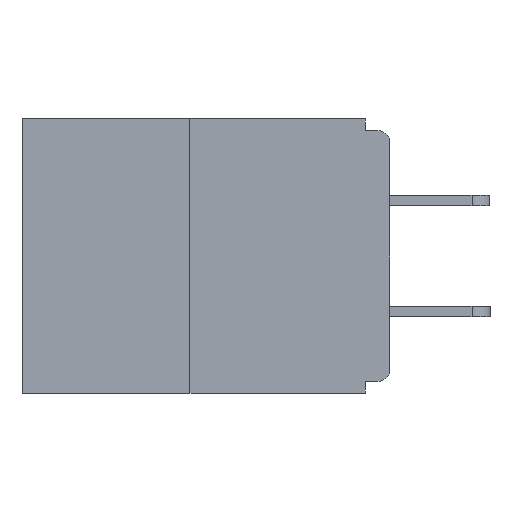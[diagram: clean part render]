
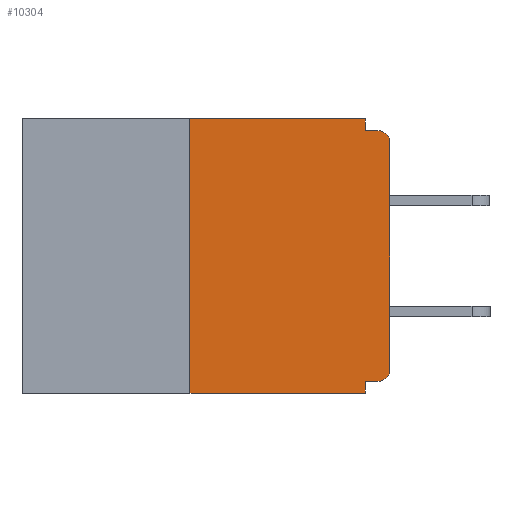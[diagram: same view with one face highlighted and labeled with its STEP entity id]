
A CAD part, left-side view. The second image highlights one B-rep face of the part: STEP entity #10304.
In plain terms, the highlighted planar face has unit normal (-1, 0, 0).
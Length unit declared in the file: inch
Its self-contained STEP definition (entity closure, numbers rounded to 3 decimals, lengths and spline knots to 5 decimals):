
#172 = CARTESIAN_POINT ( 'NONE',  ( 0., 0.25, 0. ) ) ;
#499 = EDGE_CURVE ( 'NONE', #18457, #21759, #11031, .T. ) ;
#586 = CARTESIAN_POINT ( 'NONE',  ( 0., 0.031, 0. ) ) ;
#733 = ORIENTED_EDGE ( 'NONE', *, *, #3186, .T. ) ;
#910 = LINE ( 'NONE', #6174, #18029 ) ;
#940 = DIRECTION ( 'NONE',  ( 0., -1., 0. ) ) ;
#1037 = VERTEX_POINT ( 'NONE', #5647 ) ;
#1962 = LINE ( 'NONE', #22350, #12063 ) ;
#1968 = VERTEX_POINT ( 'NONE', #5962 ) ;
#2229 = CARTESIAN_POINT ( 'NONE',  ( 0., 0.25, -0.343 ) ) ;
#3124 = EDGE_CURVE ( 'NONE', #4434, #1037, #19888, .T. ) ;
#3186 = EDGE_CURVE ( 'NONE', #19924, #1037, #22337, .T. ) ;
#3203 = ORIENTED_EDGE ( 'NONE', *, *, #18955, .T. ) ;
#3213 = CARTESIAN_POINT ( 'NONE',  ( 0., 0.015, -0.015 ) ) ;
#3236 = CARTESIAN_POINT ( 'NONE',  ( 0., 0.46, 0. ) ) ;
#3312 = ORIENTED_EDGE ( 'NONE', *, *, #21635, .F. ) ;
#3404 = CARTESIAN_POINT ( 'NONE',  ( 0., 0.031, 0. ) ) ;
#3610 = DIRECTION ( 'NONE',  ( 0., 0., -1. ) ) ;
#3666 = DIRECTION ( 'NONE',  ( 0., 0., 1. ) ) ;
#4434 = VERTEX_POINT ( 'NONE', #6158 ) ;
#4980 = DIRECTION ( 'NONE',  ( 0., 0., 1. ) ) ;
#5052 = DIRECTION ( 'NONE',  ( 0., 0., -1. ) ) ;
#5203 = DIRECTION ( 'NONE',  ( 0., 0., -1. ) ) ;
#5257 = CARTESIAN_POINT ( 'NONE',  ( 0., 0.015, -0.313 ) ) ;
#5304 = CARTESIAN_POINT ( 'NONE',  ( 0., 0.031, -0.015 ) ) ;
#5647 = CARTESIAN_POINT ( 'NONE',  ( 0., 0.031, -0.343 ) ) ;
#5962 = CARTESIAN_POINT ( 'NONE',  ( 0., 0., -0.313 ) ) ;
#6158 = CARTESIAN_POINT ( 'NONE',  ( 0., 0.031, -0.328 ) ) ;
#6174 = CARTESIAN_POINT ( 'NONE',  ( 0., 0., -0.015 ) ) ;
#6202 = EDGE_CURVE ( 'NONE', #12176, #1968, #8541, .T. ) ;
#6522 = DIRECTION ( 'NONE',  ( -1., 0., 0. ) ) ;
#7012 = CARTESIAN_POINT ( 'NONE',  ( 0., 0., -0.03 ) ) ;
#7045 = DIRECTION ( 'NONE',  ( 1., 0., 0. ) ) ;
#8274 = EDGE_LOOP ( 'NONE', ( #14241, #15948, #733, #13945, #16941, #13226, #18513, #3203, #3312, #21714 ) ) ;
#8541 = CIRCLE ( 'NONE', #15585, 0.015 ) ;
#9002 = VECTOR ( 'NONE', #3666, 39.37008 ) ;
#9113 = VECTOR ( 'NONE', #12593, 39.37008 ) ;
#9220 = FACE_OUTER_BOUND ( 'NONE', #8274, .T. ) ;
#9306 = VECTOR ( 'NONE', #5203, 39.37008 ) ;
#9502 = CARTESIAN_POINT ( 'NONE',  ( 0., 0.46, -0.343 ) ) ;
#10304 = ADVANCED_FACE ( 'NONE', ( #9220 ), #11923, .F. ) ;
#10597 = VERTEX_POINT ( 'NONE', #7012 ) ;
#10696 = LINE ( 'NONE', #15872, #16679 ) ;
#11031 = LINE ( 'NONE', #586, #9113 ) ;
#11128 = CIRCLE ( 'NONE', #17450, 0.015 ) ;
#11409 = DIRECTION ( 'NONE',  ( 0., -1., 0. ) ) ;
#11770 = CARTESIAN_POINT ( 'NONE',  ( 0., 0., 0. ) ) ;
#11923 = PLANE ( 'NONE',  #18122 ) ;
#12063 = VECTOR ( 'NONE', #12115, 39.37008 ) ;
#12115 = DIRECTION ( 'NONE',  ( 0., 1., 0. ) ) ;
#12176 = VERTEX_POINT ( 'NONE', #12956 ) ;
#12491 = CARTESIAN_POINT ( 'NONE',  ( 0., 0.25, 0. ) ) ;
#12593 = DIRECTION ( 'NONE',  ( 0., 0., -1. ) ) ;
#12677 = LINE ( 'NONE', #11770, #20739 ) ;
#12759 = EDGE_CURVE ( 'NONE', #19924, #14581, #20939, .T. ) ;
#12956 = CARTESIAN_POINT ( 'NONE',  ( 0., 0.015, -0.328 ) ) ;
#13226 = ORIENTED_EDGE ( 'NONE', *, *, #6202, .T. ) ;
#13945 = ORIENTED_EDGE ( 'NONE', *, *, #3124, .F. ) ;
#14241 = ORIENTED_EDGE ( 'NONE', *, *, #18108, .F. ) ;
#14581 = VERTEX_POINT ( 'NONE', #12491 ) ;
#15316 = CARTESIAN_POINT ( 'NONE',  ( 0., 0.015, -0.03 ) ) ;
#15585 = AXIS2_PLACEMENT_3D ( 'NONE', #5257, #15679, #17448 ) ;
#15679 = DIRECTION ( 'NONE',  ( -1., 0., 0. ) ) ;
#15872 = CARTESIAN_POINT ( 'NONE',  ( 0., 0.46, 0. ) ) ;
#15948 = ORIENTED_EDGE ( 'NONE', *, *, #12759, .F. ) ;
#16679 = VECTOR ( 'NONE', #17856, 39.37008 ) ;
#16941 = ORIENTED_EDGE ( 'NONE', *, *, #21707, .F. ) ;
#17448 = DIRECTION ( 'NONE',  ( 0., 0., -1. ) ) ;
#17450 = AXIS2_PLACEMENT_3D ( 'NONE', #15316, #6522, #5052 ) ;
#17608 = CARTESIAN_POINT ( 'NONE',  ( 0., 0.031, -0.343 ) ) ;
#17856 = DIRECTION ( 'NONE',  ( 0., -1., 0. ) ) ;
#18029 = VECTOR ( 'NONE', #11409, 39.37008 ) ;
#18108 = EDGE_CURVE ( 'NONE', #14581, #18457, #10696, .T. ) ;
#18122 = AXIS2_PLACEMENT_3D ( 'NONE', #3236, #7045, #3610 ) ;
#18457 = VERTEX_POINT ( 'NONE', #3404 ) ;
#18513 = ORIENTED_EDGE ( 'NONE', *, *, #18960, .T. ) ;
#18955 = EDGE_CURVE ( 'NONE', #10597, #22397, #11128, .T. ) ;
#18960 = EDGE_CURVE ( 'NONE', #1968, #10597, #12677, .T. ) ;
#19888 = LINE ( 'NONE', #17608, #9306 ) ;
#19924 = VERTEX_POINT ( 'NONE', #2229 ) ;
#20167 = VECTOR ( 'NONE', #940, 39.37008 ) ;
#20739 = VECTOR ( 'NONE', #4980, 39.37008 ) ;
#20939 = LINE ( 'NONE', #172, #9002 ) ;
#21635 = EDGE_CURVE ( 'NONE', #21759, #22397, #910, .T. ) ;
#21707 = EDGE_CURVE ( 'NONE', #12176, #4434, #1962, .T. ) ;
#21714 = ORIENTED_EDGE ( 'NONE', *, *, #499, .F. ) ;
#21759 = VERTEX_POINT ( 'NONE', #5304 ) ;
#22337 = LINE ( 'NONE', #9502, #20167 ) ;
#22350 = CARTESIAN_POINT ( 'NONE',  ( 0., 0., -0.328 ) ) ;
#22397 = VERTEX_POINT ( 'NONE', #3213 ) ;
